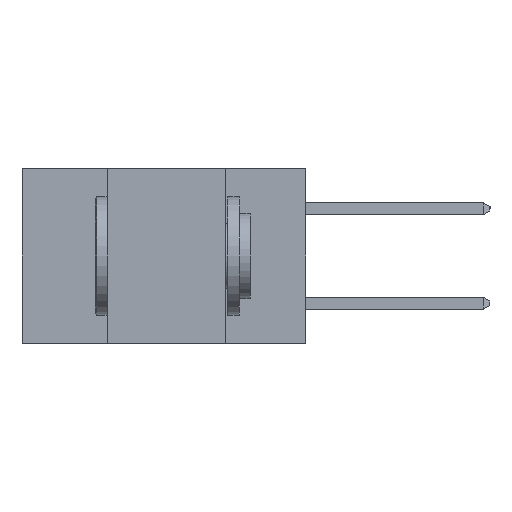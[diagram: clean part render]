
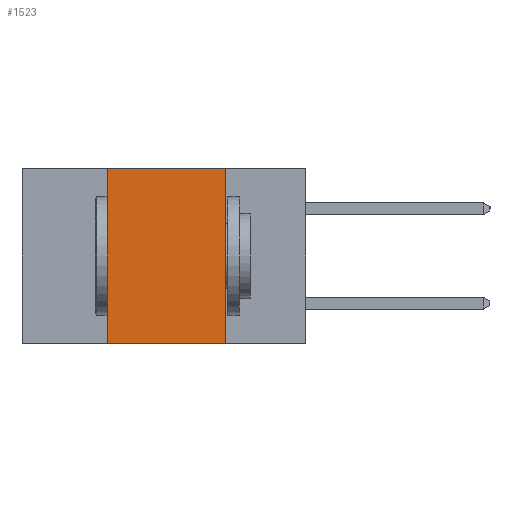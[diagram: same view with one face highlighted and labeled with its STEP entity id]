
A CAD part, left-side view. The second image highlights one B-rep face of the part: STEP entity #1523.
In plain terms, the highlighted planar face has unit normal (-1, 0, 0).
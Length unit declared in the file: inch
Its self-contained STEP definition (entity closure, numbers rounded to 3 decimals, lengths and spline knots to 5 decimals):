
#1523 = ADVANCED_FACE ( 'NONE', ( #5159 ), #2373, .F. ) ;
#1596 = VECTOR ( 'NONE', #16739, 39.37008 ) ;
#1776 = LINE ( 'NONE', #15123, #3138 ) ;
#2155 = CARTESIAN_POINT ( 'NONE',  ( 0., 0.42, 0. ) ) ;
#2373 = PLANE ( 'NONE',  #13950 ) ;
#2562 = VECTOR ( 'NONE', #17197, 39.37008 ) ;
#2893 = LINE ( 'NONE', #18224, #1596 ) ;
#3138 = VECTOR ( 'NONE', #6041, 39.37008 ) ;
#4176 = LINE ( 'NONE', #16346, #16784 ) ;
#5159 = FACE_OUTER_BOUND ( 'NONE', #6548, .T. ) ;
#5593 = VERTEX_POINT ( 'NONE', #15748 ) ;
#5969 = VERTEX_POINT ( 'NONE', #9639 ) ;
#6041 = DIRECTION ( 'NONE',  ( 0., -1., 0. ) ) ;
#6346 = EDGE_CURVE ( 'NONE', #15017, #5969, #1776, .T. ) ;
#6548 = EDGE_LOOP ( 'NONE', ( #18922, #13507, #6589, #10933 ) ) ;
#6589 = ORIENTED_EDGE ( 'NONE', *, *, #18183, .F. ) ;
#6749 = CARTESIAN_POINT ( 'NONE',  ( 0., 0.6, 0. ) ) ;
#7886 = VERTEX_POINT ( 'NONE', #2155 ) ;
#8568 = CARTESIAN_POINT ( 'NONE',  ( 0., 0.42, -0.37 ) ) ;
#9639 = CARTESIAN_POINT ( 'NONE',  ( 0., 0.17, -0.37 ) ) ;
#10933 = ORIENTED_EDGE ( 'NONE', *, *, #6346, .T. ) ;
#11129 = CARTESIAN_POINT ( 'NONE',  ( 0., 0.17, -0.37 ) ) ;
#12829 = DIRECTION ( 'NONE',  ( 1., 0., 0. ) ) ;
#13507 = ORIENTED_EDGE ( 'NONE', *, *, #13900, .F. ) ;
#13900 = EDGE_CURVE ( 'NONE', #7886, #5593, #4176, .T. ) ;
#13950 = AXIS2_PLACEMENT_3D ( 'NONE', #6749, #12829, #15908 ) ;
#15017 = VERTEX_POINT ( 'NONE', #8568 ) ;
#15123 = CARTESIAN_POINT ( 'NONE',  ( 0., 0.6, -0.37 ) ) ;
#15705 = DIRECTION ( 'NONE',  ( 0., -1., 0. ) ) ;
#15748 = CARTESIAN_POINT ( 'NONE',  ( 0., 0.17, 0. ) ) ;
#15809 = LINE ( 'NONE', #11129, #2562 ) ;
#15908 = DIRECTION ( 'NONE',  ( 0., 0., -1. ) ) ;
#16346 = CARTESIAN_POINT ( 'NONE',  ( 0., 0.6, 0. ) ) ;
#16739 = DIRECTION ( 'NONE',  ( 0., 0., 1. ) ) ;
#16784 = VECTOR ( 'NONE', #15705, 39.37008 ) ;
#17197 = DIRECTION ( 'NONE',  ( 0., 0., -1. ) ) ;
#18183 = EDGE_CURVE ( 'NONE', #15017, #7886, #2893, .T. ) ;
#18224 = CARTESIAN_POINT ( 'NONE',  ( 0., 0.42, -0.37 ) ) ;
#18881 = EDGE_CURVE ( 'NONE', #5593, #5969, #15809, .T. ) ;
#18922 = ORIENTED_EDGE ( 'NONE', *, *, #18881, .F. ) ;
